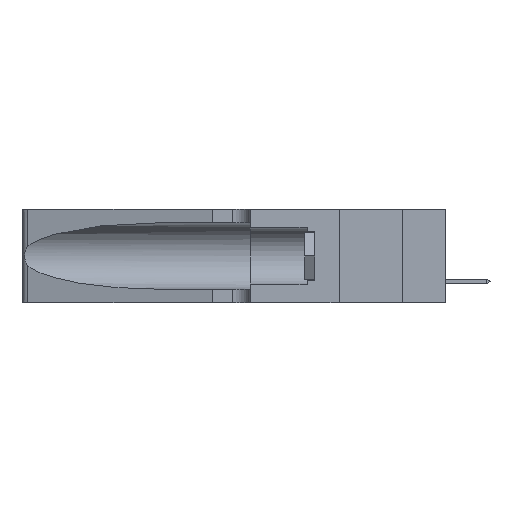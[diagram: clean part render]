
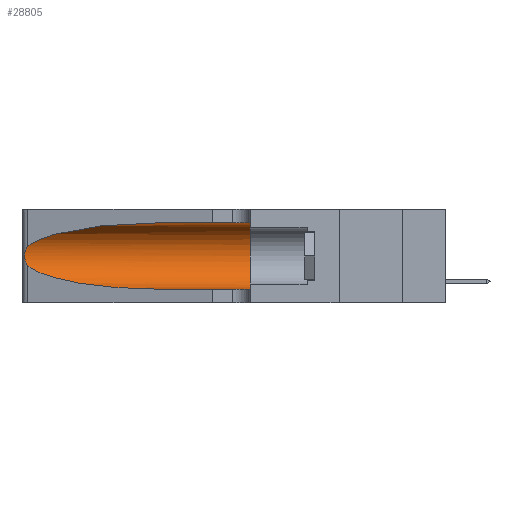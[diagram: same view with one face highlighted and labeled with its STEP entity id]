
A CAD part, left-side view. The second image highlights one B-rep face of the part: STEP entity #28805.
In plain terms, the highlighted cylindrical face has radius 3.308 mm (diameter 6.617 mm), a partial arc.
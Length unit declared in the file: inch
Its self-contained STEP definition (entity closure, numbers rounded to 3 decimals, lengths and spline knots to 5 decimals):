
#482 =( BOUNDED_CURVE ( )  B_SPLINE_CURVE ( 3, ( #32442, #40453, #28811, #48941 ),
 .UNSPECIFIED., .F., .F. ) 
 B_SPLINE_CURVE_WITH_KNOTS ( ( 4, 4 ),
 ( 3.44316, 4.71239 ),
 .UNSPECIFIED. ) 
 CURVE ( )  GEOMETRIC_REPRESENTATION_ITEM ( )  RATIONAL_B_SPLINE_CURVE ( ( 1., 0.87, 0.87, 1. ) ) 
 REPRESENTATION_ITEM ( '' )  );
#1245 = EDGE_CURVE ( 'NONE', #8769, #44309, #28058, .T. ) ;
#1415 = DIRECTION ( 'NONE',  ( 0., -1., 0. ) ) ;
#3131 = CARTESIAN_POINT ( 'NONE',  ( 0.25555, 1.22993, 0.14849 ) ) ;
#3647 = DIRECTION ( 'NONE',  ( 0., 0., -1. ) ) ;
#3873 = CARTESIAN_POINT ( 'NONE',  ( 0.25487, 1.22718, 0.22369 ) ) ;
#3928 = LINE ( 'NONE', #21092, #18772 ) ;
#4907 =( BOUNDED_CURVE ( )  B_SPLINE_CURVE ( 3, ( #31193, #26870, #35200, #3873 ),
 .UNSPECIFIED., .F., .T. ) 
 B_SPLINE_CURVE_WITH_KNOTS ( ( 4, 4 ),
 ( 1.5708, 2.84003 ),
 .UNSPECIFIED. ) 
 CURVE ( )  GEOMETRIC_REPRESENTATION_ITEM ( )  RATIONAL_B_SPLINE_CURVE ( ( 1., 0.87, 0.87, 1. ) ) 
 REPRESENTATION_ITEM ( '' )  );
#5643 = CARTESIAN_POINT ( 'NONE',  ( 0.1305, 0.35, 0.31525 ) ) ;
#7013 = FACE_OUTER_BOUND ( 'NONE', #42066, .T. ) ;
#7126 = ORIENTED_EDGE ( 'NONE', *, *, #44508, .T. ) ;
#7830 = CARTESIAN_POINT ( 'NONE',  ( 0.1305, 1.61858, 0.05475 ) ) ;
#8769 = VERTEX_POINT ( 'NONE', #5643 ) ;
#9021 = CARTESIAN_POINT ( 'NONE',  ( 0.1305, 0.72297, 0.05475 ) ) ;
#9664 = B_SPLINE_CURVE_WITH_KNOTS ( 'NONE', 3,
 ( #18480, #30417, #11065, #41877, #46572, #34076, #46418, #14505, #38578, #50537, #22777, #26764, #3131, #34600 ),
 .UNSPECIFIED., .F., .F.,
 ( 4, 2, 2, 2, 2, 2, 4 ),
 ( 0., 0.00027, 0.00053, 0.00107, 0.0016, 0.00187, 0.00214 ),
 .UNSPECIFIED. ) ;
#10759 = DIRECTION ( 'NONE',  ( 0., -1., 0. ) ) ;
#11065 = CARTESIAN_POINT ( 'NONE',  ( 0.25639, 1.23184, 0.21858 ) ) ;
#13661 = ORIENTED_EDGE ( 'NONE', *, *, #46240, .T. ) ;
#14125 = VERTEX_POINT ( 'NONE', #40024 ) ;
#14306 = VERTEX_POINT ( 'NONE', #9021 ) ;
#14505 = CARTESIAN_POINT ( 'NONE',  ( 0.26075, 1.23896, 0.178 ) ) ;
#15042 = CARTESIAN_POINT ( 'NONE',  ( 0.25487, 1.22718, 0.14631 ) ) ;
#16570 = VERTEX_POINT ( 'NONE', #48757 ) ;
#18480 = CARTESIAN_POINT ( 'NONE',  ( 0.25487, 1.22718, 0.22369 ) ) ;
#18772 = VECTOR ( 'NONE', #1415, 39.37008 ) ;
#21092 = CARTESIAN_POINT ( 'NONE',  ( 0.1305, 1.61858, 0.31525 ) ) ;
#22777 = CARTESIAN_POINT ( 'NONE',  ( 0.25789, 1.23486, 0.15765 ) ) ;
#23881 = ORIENTED_EDGE ( 'NONE', *, *, #39665, .F. ) ;
#25169 = ORIENTED_EDGE ( 'NONE', *, *, #43374, .T. ) ;
#25848 = ORIENTED_EDGE ( 'NONE', *, *, #1245, .F. ) ;
#26672 = DIRECTION ( 'NONE',  ( 0., 0., 1. ) ) ;
#26764 = CARTESIAN_POINT ( 'NONE',  ( 0.25639, 1.23186, 0.15144 ) ) ;
#26870 = CARTESIAN_POINT ( 'NONE',  ( 0.18966, 0.96281, 0.31525 ) ) ;
#28058 = CIRCLE ( 'NONE', #45550, 0.13025 ) ;
#28805 = ADVANCED_FACE ( 'NONE', ( #7013 ), #49724, .F. ) ;
#28811 = CARTESIAN_POINT ( 'NONE',  ( 0.18966, 0.96281, 0.05475 ) ) ;
#28851 = LINE ( 'NONE', #7830, #36926 ) ;
#29291 = CARTESIAN_POINT ( 'NONE',  ( 0.1305, 0.35, 0.05475 ) ) ;
#30417 = CARTESIAN_POINT ( 'NONE',  ( 0.25555, 1.22994, 0.2215 ) ) ;
#31193 = CARTESIAN_POINT ( 'NONE',  ( 0.1305, 0.72297, 0.31525 ) ) ;
#32442 = CARTESIAN_POINT ( 'NONE',  ( 0.25487, 1.22718, 0.14631 ) ) ;
#32746 = AXIS2_PLACEMENT_3D ( 'NONE', #42593, #10759, #3647 ) ;
#34076 = CARTESIAN_POINT ( 'NONE',  ( 0.26018, 1.23835, 0.19895 ) ) ;
#34600 = CARTESIAN_POINT ( 'NONE',  ( 0.25487, 1.22718, 0.14631 ) ) ;
#34662 = CARTESIAN_POINT ( 'NONE',  ( 0.1305, 0.35, 0.185 ) ) ;
#35200 = CARTESIAN_POINT ( 'NONE',  ( 0.2373, 1.15595, 0.28018 ) ) ;
#35293 = VERTEX_POINT ( 'NONE', #15042 ) ;
#36926 = VECTOR ( 'NONE', #46956, 39.37008 ) ;
#37628 = ORIENTED_EDGE ( 'NONE', *, *, #46468, .T. ) ;
#38578 = CARTESIAN_POINT ( 'NONE',  ( 0.26017, 1.23833, 0.17102 ) ) ;
#39665 = EDGE_CURVE ( 'NONE', #14125, #8769, #3928, .T. ) ;
#40024 = CARTESIAN_POINT ( 'NONE',  ( 0.1305, 0.72297, 0.31525 ) ) ;
#40453 = CARTESIAN_POINT ( 'NONE',  ( 0.2373, 1.15595, 0.08982 ) ) ;
#41877 = CARTESIAN_POINT ( 'NONE',  ( 0.25787, 1.23484, 0.2124 ) ) ;
#42066 = EDGE_LOOP ( 'NONE', ( #7126, #13661, #37628, #25169, #25848, #23881 ) ) ;
#42593 = CARTESIAN_POINT ( 'NONE',  ( 0.1305, 1.61858, 0.185 ) ) ;
#43374 = EDGE_CURVE ( 'NONE', #14306, #44309, #28851, .T. ) ;
#44309 = VERTEX_POINT ( 'NONE', #29291 ) ;
#44508 = EDGE_CURVE ( 'NONE', #14125, #16570, #4907, .T. ) ;
#45550 = AXIS2_PLACEMENT_3D ( 'NONE', #34662, #50427, #26672 ) ;
#46240 = EDGE_CURVE ( 'NONE', #16570, #35293, #9664, .T. ) ;
#46418 = CARTESIAN_POINT ( 'NONE',  ( 0.26075, 1.23896, 0.19203 ) ) ;
#46468 = EDGE_CURVE ( 'NONE', #35293, #14306, #482, .T. ) ;
#46572 = CARTESIAN_POINT ( 'NONE',  ( 0.25854, 1.2359, 0.20912 ) ) ;
#46956 = DIRECTION ( 'NONE',  ( 0., -1., 0. ) ) ;
#48757 = CARTESIAN_POINT ( 'NONE',  ( 0.25487, 1.22718, 0.22369 ) ) ;
#48941 = CARTESIAN_POINT ( 'NONE',  ( 0.1305, 0.72297, 0.05475 ) ) ;
#49724 = CYLINDRICAL_SURFACE ( 'NONE', #32746, 0.13025 ) ;
#50427 = DIRECTION ( 'NONE',  ( 0., 1., 0. ) ) ;
#50537 = CARTESIAN_POINT ( 'NONE',  ( 0.25856, 1.23593, 0.16098 ) ) ;
